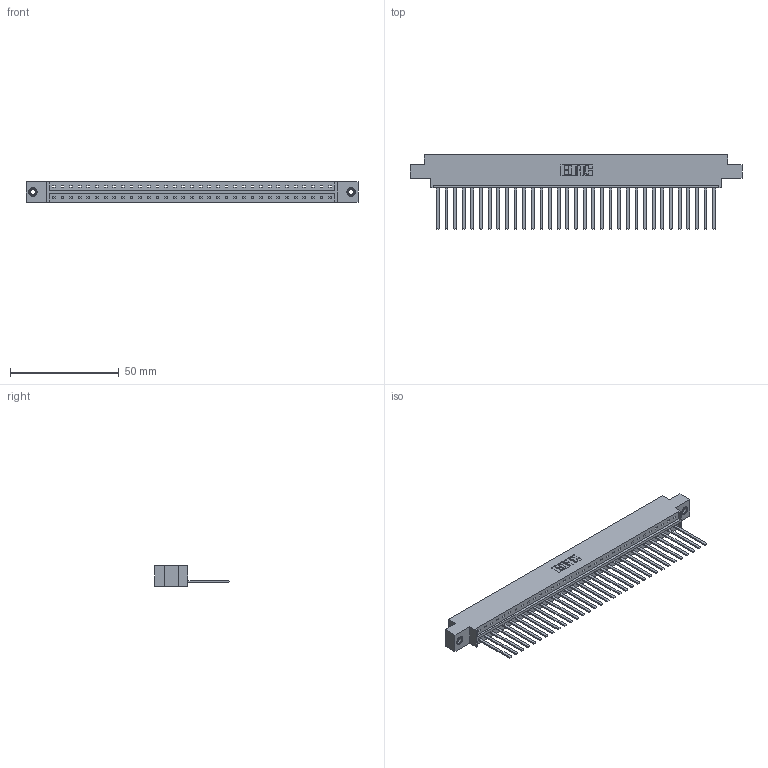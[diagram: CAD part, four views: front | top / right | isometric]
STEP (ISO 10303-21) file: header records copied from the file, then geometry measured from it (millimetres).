
FILE_DESCRIPTION (( 'STEP AP203' ), '1' );
FILE_NAME ('333-033-544-608.STEP', '2018-08-02T21:26:53', ( '' ), ( '' ), 'SwSTEP 2.0', 'SolidWorks 2016', '' );
FILE_SCHEMA (( 'CONFIG_CONTROL_DESIGN' ));
Length unit declared in the file: inch
Products named in the file (4): 333-033-544-608; 333 Part_Offset - .156 Dia - TI; 345-292-001_345-293-144; 345-250-001_345-250-003-102
Assembly tree (36 placements, depth 2):
  333-033-544-608
    333 Part_Offset - .156 Dia - TI
    345-292-001_345-293-144  x33
    345-250-001_345-250-003-102  x2
Bounding box: 152.3 x 34.3 x 9.4 mm (x, y, z)
Volume: 15396 mm3; surface area: 18065.9 mm2
Topology: 36 solids, 36 shells, 1894 faces, 5673 edges, 3730 vertices
Faces by surface type: plane 1360, cylinder 518, cone 12, torus 4
Entity records: 22472 total; most frequent: CARTESIAN_POINT 3860, ORIENTED_EDGE 3822, DIRECTION 3303, EDGE_CURVE 1911, VECTOR 1767, LINE 1767, VERTEX_POINT 1268, AXIS2_PLACEMENT_3D 768
